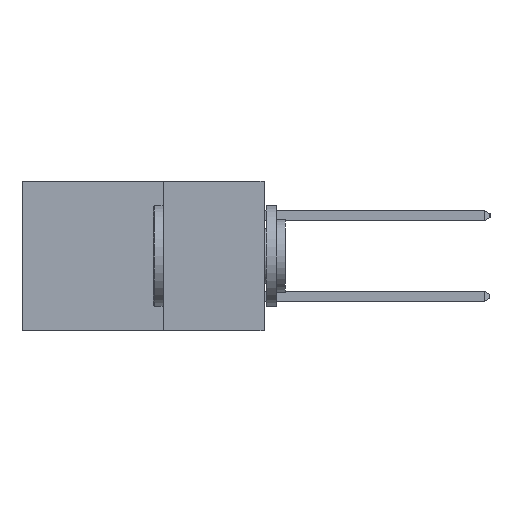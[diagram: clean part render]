
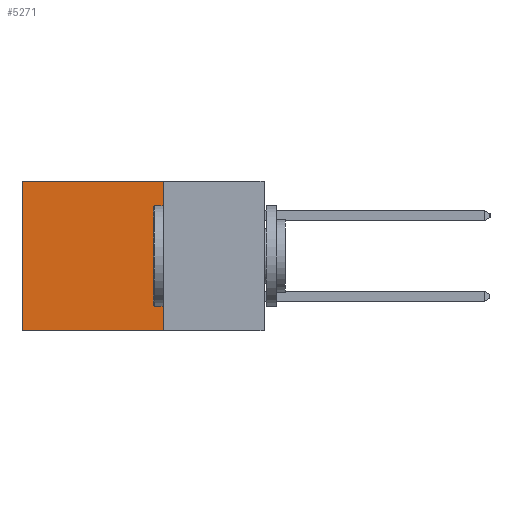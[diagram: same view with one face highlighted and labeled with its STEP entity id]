
A CAD part, left-side view. The second image highlights one B-rep face of the part: STEP entity #5271.
In plain terms, the highlighted planar face has unit normal (-1, 0, 0).
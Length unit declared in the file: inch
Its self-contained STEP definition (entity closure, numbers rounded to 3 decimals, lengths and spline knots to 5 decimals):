
#750 = CARTESIAN_POINT ( 'NONE',  ( 0.2615, 0.25, -0.37 ) ) ;
#2574 = CARTESIAN_POINT ( 'NONE',  ( 0.2615, 0.6, -0.37 ) ) ;
#4958 = VERTEX_POINT ( 'NONE', #20321 ) ;
#5167 = VERTEX_POINT ( 'NONE', #19061 ) ;
#5271 = ADVANCED_FACE ( 'NONE', ( #26054 ), #6829, .F. ) ;
#6239 = CARTESIAN_POINT ( 'NONE',  ( 0.2615, 0.25, -0.37 ) ) ;
#6687 = CARTESIAN_POINT ( 'NONE',  ( 0.2615, 0.6, 0. ) ) ;
#6829 = PLANE ( 'NONE',  #20122 ) ;
#6955 = VECTOR ( 'NONE', #19975, 39.37008 ) ;
#7711 = DIRECTION ( 'NONE',  ( 0., 1., 0. ) ) ;
#11933 = LINE ( 'NONE', #18392, #15677 ) ;
#12565 = ORIENTED_EDGE ( 'NONE', *, *, #14941, .F. ) ;
#13027 = ORIENTED_EDGE ( 'NONE', *, *, #15423, .T. ) ;
#13220 = VECTOR ( 'NONE', #26177, 39.37008 ) ;
#13848 = VECTOR ( 'NONE', #26567, 39.37008 ) ;
#14941 = EDGE_CURVE ( 'NONE', #4958, #25455, #25913, .T. ) ;
#15016 = DIRECTION ( 'NONE',  ( 1., 0., 0. ) ) ;
#15285 = DIRECTION ( 'NONE',  ( 0., 0., -1. ) ) ;
#15423 = EDGE_CURVE ( 'NONE', #22163, #5167, #25885, .T. ) ;
#15677 = VECTOR ( 'NONE', #7711, 39.37008 ) ;
#16763 = ORIENTED_EDGE ( 'NONE', *, *, #23325, .T. ) ;
#18392 = CARTESIAN_POINT ( 'NONE',  ( 0.2615, 0.25, 0. ) ) ;
#19061 = CARTESIAN_POINT ( 'NONE',  ( 0.2615, 0.6, -0.37 ) ) ;
#19975 = DIRECTION ( 'NONE',  ( 0., 0., -1. ) ) ;
#20122 = AXIS2_PLACEMENT_3D ( 'NONE', #21842, #15016, #15285 ) ;
#20321 = CARTESIAN_POINT ( 'NONE',  ( 0.2615, 0.25, 0. ) ) ;
#21842 = CARTESIAN_POINT ( 'NONE',  ( 0.2615, 0.25, -0.37 ) ) ;
#22102 = CARTESIAN_POINT ( 'NONE',  ( 0.2615, 0.25, -0.37 ) ) ;
#22163 = VERTEX_POINT ( 'NONE', #6687 ) ;
#22685 = EDGE_CURVE ( 'NONE', #25455, #5167, #26287, .T. ) ;
#22933 = ORIENTED_EDGE ( 'NONE', *, *, #22685, .F. ) ;
#23325 = EDGE_CURVE ( 'NONE', #4958, #22163, #11933, .T. ) ;
#24331 = EDGE_LOOP ( 'NONE', ( #13027, #22933, #12565, #16763 ) ) ;
#25455 = VERTEX_POINT ( 'NONE', #6239 ) ;
#25885 = LINE ( 'NONE', #2574, #6955 ) ;
#25913 = LINE ( 'NONE', #22102, #13220 ) ;
#26054 = FACE_OUTER_BOUND ( 'NONE', #24331, .T. ) ;
#26177 = DIRECTION ( 'NONE',  ( 0., 0., -1. ) ) ;
#26287 = LINE ( 'NONE', #750, #13848 ) ;
#26567 = DIRECTION ( 'NONE',  ( 0., 1., 0. ) ) ;
